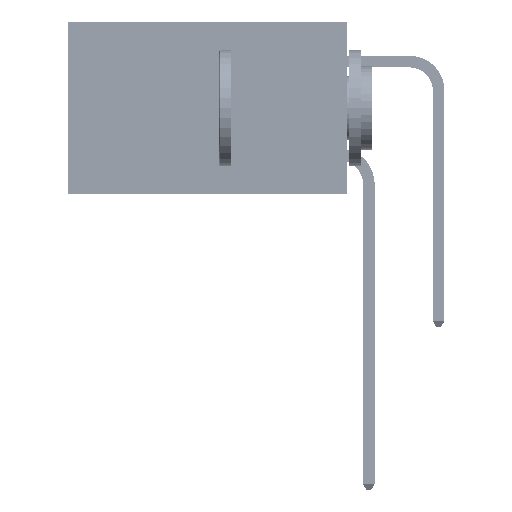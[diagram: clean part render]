
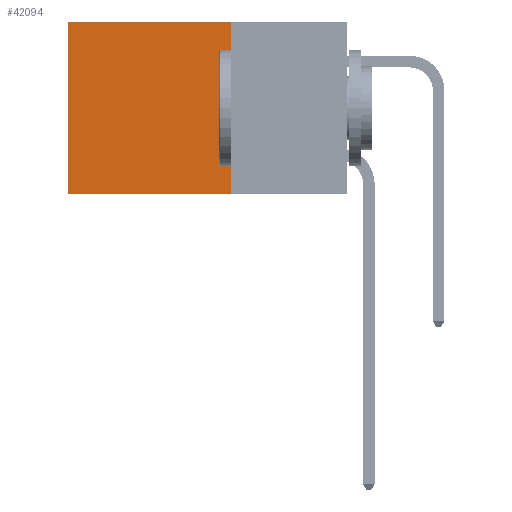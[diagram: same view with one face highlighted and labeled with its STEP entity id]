
A CAD part, left-side view. The second image highlights one B-rep face of the part: STEP entity #42094.
In plain terms, the highlighted planar face has unit normal (-1, 0, 0).
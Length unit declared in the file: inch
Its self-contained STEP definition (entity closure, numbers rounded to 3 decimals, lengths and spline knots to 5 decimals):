
#572 = DIRECTION ( 'NONE',  ( 1., 0., 0. ) ) ;
#884 = VECTOR ( 'NONE', #5462, 39.37008 ) ;
#1333 = DIRECTION ( 'NONE',  ( 0., 1., 0. ) ) ;
#1746 = CARTESIAN_POINT ( 'NONE',  ( 0.2875, 0.6, 0. ) ) ;
#1882 = ORIENTED_EDGE ( 'NONE', *, *, #34838, .T. ) ;
#5462 = DIRECTION ( 'NONE',  ( 0., 1., 0. ) ) ;
#12761 = LINE ( 'NONE', #1746, #40814 ) ;
#12807 = VERTEX_POINT ( 'NONE', #18726 ) ;
#13028 = CARTESIAN_POINT ( 'NONE',  ( 0.2875, 0.25, 0. ) ) ;
#13603 = CARTESIAN_POINT ( 'NONE',  ( 0.2875, 0.25, 0. ) ) ;
#15547 = CARTESIAN_POINT ( 'NONE',  ( 0.2875, 0.25, 0. ) ) ;
#16165 = AXIS2_PLACEMENT_3D ( 'NONE', #15547, #572, #26701 ) ;
#17360 = DIRECTION ( 'NONE',  ( 0., 0., -1. ) ) ;
#18726 = CARTESIAN_POINT ( 'NONE',  ( 0.2875, 0.25, 0. ) ) ;
#19222 = ORIENTED_EDGE ( 'NONE', *, *, #41935, .F. ) ;
#20031 = CARTESIAN_POINT ( 'NONE',  ( 0.2875, 0.25, -0.37 ) ) ;
#21904 = FACE_OUTER_BOUND ( 'NONE', #37360, .T. ) ;
#23529 = CARTESIAN_POINT ( 'NONE',  ( 0.2875, 0.6, -0.37 ) ) ;
#26060 = EDGE_CURVE ( 'NONE', #44883, #28064, #12761, .T. ) ;
#26701 = DIRECTION ( 'NONE',  ( 0., 0., -1. ) ) ;
#28064 = VERTEX_POINT ( 'NONE', #23529 ) ;
#28098 = VECTOR ( 'NONE', #17360, 39.37008 ) ;
#28143 = EDGE_CURVE ( 'NONE', #12807, #30807, #29205, .T. ) ;
#28770 = VECTOR ( 'NONE', #1333, 39.37008 ) ;
#29205 = LINE ( 'NONE', #13603, #28098 ) ;
#30807 = VERTEX_POINT ( 'NONE', #33156 ) ;
#31050 = LINE ( 'NONE', #20031, #28770 ) ;
#33156 = CARTESIAN_POINT ( 'NONE',  ( 0.2875, 0.25, -0.37 ) ) ;
#34315 = ORIENTED_EDGE ( 'NONE', *, *, #28143, .F. ) ;
#34838 = EDGE_CURVE ( 'NONE', #12807, #44883, #41332, .T. ) ;
#37360 = EDGE_LOOP ( 'NONE', ( #43206, #19222, #34315, #1882 ) ) ;
#37486 = PLANE ( 'NONE',  #16165 ) ;
#38760 = DIRECTION ( 'NONE',  ( 0., 0., -1. ) ) ;
#40814 = VECTOR ( 'NONE', #38760, 39.37008 ) ;
#41332 = LINE ( 'NONE', #13028, #884 ) ;
#41935 = EDGE_CURVE ( 'NONE', #30807, #28064, #31050, .T. ) ;
#42094 = ADVANCED_FACE ( 'NONE', ( #21904 ), #37486, .F. ) ;
#43206 = ORIENTED_EDGE ( 'NONE', *, *, #26060, .T. ) ;
#44883 = VERTEX_POINT ( 'NONE', #46032 ) ;
#46032 = CARTESIAN_POINT ( 'NONE',  ( 0.2875, 0.6, 0. ) ) ;
